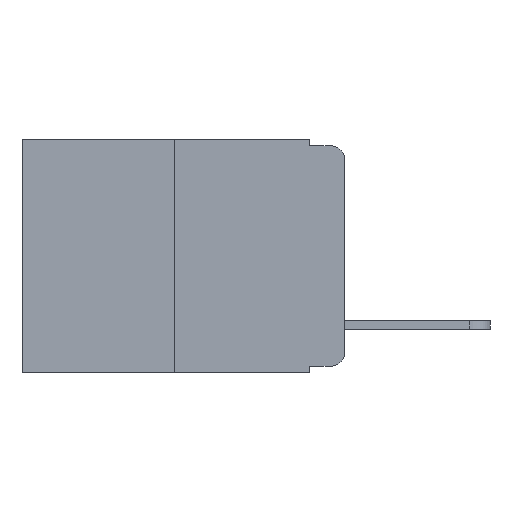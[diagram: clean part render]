
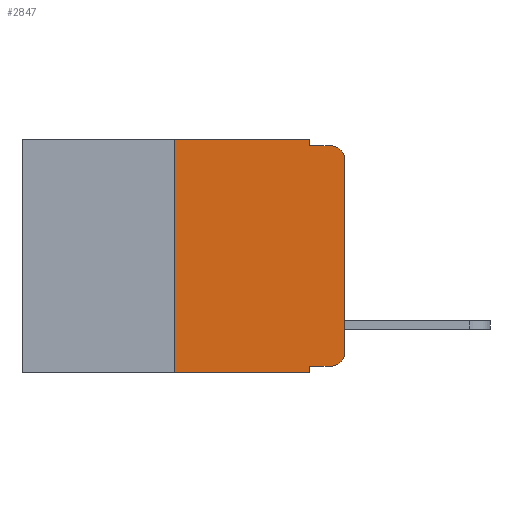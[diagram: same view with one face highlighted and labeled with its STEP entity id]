
A CAD part, left-side view. The second image highlights one B-rep face of the part: STEP entity #2847.
In plain terms, the highlighted planar face has unit normal (-1, 0, 0).
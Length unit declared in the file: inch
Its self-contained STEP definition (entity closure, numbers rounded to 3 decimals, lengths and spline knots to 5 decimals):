
#247 = PLANE ( 'NONE',  #12645 ) ;
#307 = DIRECTION ( 'NONE',  ( 0., 0., -1. ) ) ;
#566 = CARTESIAN_POINT ( 'NONE',  ( 0., 0.051, 0. ) ) ;
#1475 = EDGE_CURVE ( 'NONE', #16898, #6367, #20616, .T. ) ;
#1575 = VECTOR ( 'NONE', #20858, 39.37008 ) ;
#2296 = ORIENTED_EDGE ( 'NONE', *, *, #19439, .T. ) ;
#2613 = EDGE_CURVE ( 'NONE', #16524, #15488, #7003, .T. ) ;
#2847 = ADVANCED_FACE ( 'NONE', ( #14139 ), #247, .F. ) ;
#3010 = EDGE_LOOP ( 'NONE', ( #2296, #21992, #5674, #8573, #14335, #6886, #19723, #22819, #3377, #20828 ) ) ;
#3377 = ORIENTED_EDGE ( 'NONE', *, *, #6042, .T. ) ;
#3824 = DIRECTION ( 'NONE',  ( 1., 0., 0. ) ) ;
#3899 = CARTESIAN_POINT ( 'NONE',  ( 0., 0.473, 0. ) ) ;
#4034 = AXIS2_PLACEMENT_3D ( 'NONE', #17190, #6256, #18954 ) ;
#4114 = DIRECTION ( 'NONE',  ( 0., 0., -1. ) ) ;
#4249 = CARTESIAN_POINT ( 'NONE',  ( 0., 0.25, 0. ) ) ;
#4371 = DIRECTION ( 'NONE',  ( 0., 0., -1. ) ) ;
#4599 = CARTESIAN_POINT ( 'NONE',  ( 0., 0.051, 0. ) ) ;
#4696 = CARTESIAN_POINT ( 'NONE',  ( 0., 0.02, -0.333 ) ) ;
#5012 = CARTESIAN_POINT ( 'NONE',  ( 0., 0.051, -0.333 ) ) ;
#5510 = CARTESIAN_POINT ( 'NONE',  ( 0., 0.051, -0.343 ) ) ;
#5674 = ORIENTED_EDGE ( 'NONE', *, *, #14672, .F. ) ;
#5768 = VECTOR ( 'NONE', #14262, 39.37008 ) ;
#6014 = VECTOR ( 'NONE', #16148, 39.37008 ) ;
#6042 = EDGE_CURVE ( 'NONE', #18162, #9641, #23542, .T. ) ;
#6256 = DIRECTION ( 'NONE',  ( -1., 0., 0. ) ) ;
#6362 = VECTOR ( 'NONE', #307, 39.37008 ) ;
#6367 = VERTEX_POINT ( 'NONE', #5510 ) ;
#6886 = ORIENTED_EDGE ( 'NONE', *, *, #12231, .F. ) ;
#7003 = LINE ( 'NONE', #13521, #20836 ) ;
#7691 = VECTOR ( 'NONE', #4371, 39.37008 ) ;
#8511 = EDGE_CURVE ( 'NONE', #18162, #6367, #21948, .T. ) ;
#8573 = ORIENTED_EDGE ( 'NONE', *, *, #13457, .F. ) ;
#8756 = CARTESIAN_POINT ( 'NONE',  ( 0., 0.051, 0. ) ) ;
#8866 = CARTESIAN_POINT ( 'NONE',  ( 0., 0.25, -0.343 ) ) ;
#9131 = CARTESIAN_POINT ( 'NONE',  ( 0., 0.02, -0.03 ) ) ;
#9641 = VERTEX_POINT ( 'NONE', #4696 ) ;
#9695 = CARTESIAN_POINT ( 'NONE',  ( 0., 0.051, -0.01 ) ) ;
#11039 = DIRECTION ( 'NONE',  ( 0., 0., -1. ) ) ;
#11094 = VECTOR ( 'NONE', #21853, 39.37008 ) ;
#12142 = LINE ( 'NONE', #12144, #16405 ) ;
#12144 = CARTESIAN_POINT ( 'NONE',  ( 0., 0., 0. ) ) ;
#12231 = EDGE_CURVE ( 'NONE', #16898, #16524, #20626, .T. ) ;
#12645 = AXIS2_PLACEMENT_3D ( 'NONE', #3899, #3824, #4114 ) ;
#13457 = EDGE_CURVE ( 'NONE', #15488, #18461, #21834, .T. ) ;
#13521 = CARTESIAN_POINT ( 'NONE',  ( 0., 0.473, 0. ) ) ;
#13653 = DIRECTION ( 'NONE',  ( 0., -1., 0. ) ) ;
#13975 = DIRECTION ( 'NONE',  ( 0., 0., 1. ) ) ;
#14094 = CARTESIAN_POINT ( 'NONE',  ( 0., 0.051, -0.333 ) ) ;
#14139 = FACE_OUTER_BOUND ( 'NONE', #3010, .T. ) ;
#14262 = DIRECTION ( 'NONE',  ( 0., -1., 0. ) ) ;
#14335 = ORIENTED_EDGE ( 'NONE', *, *, #2613, .F. ) ;
#14672 = EDGE_CURVE ( 'NONE', #18461, #18626, #15785, .T. ) ;
#15488 = VERTEX_POINT ( 'NONE', #8756 ) ;
#15774 = CIRCLE ( 'NONE', #4034, 0.02 ) ;
#15785 = LINE ( 'NONE', #16197, #6014 ) ;
#16148 = DIRECTION ( 'NONE',  ( 0., -1., 0. ) ) ;
#16197 = CARTESIAN_POINT ( 'NONE',  ( 0., 0.051, -0.01 ) ) ;
#16405 = VECTOR ( 'NONE', #13975, 39.37008 ) ;
#16524 = VERTEX_POINT ( 'NONE', #4249 ) ;
#16574 = CARTESIAN_POINT ( 'NONE',  ( 0., 0., -0.03 ) ) ;
#16898 = VERTEX_POINT ( 'NONE', #8866 ) ;
#17190 = CARTESIAN_POINT ( 'NONE',  ( 0., 0.02, -0.313 ) ) ;
#17440 = CARTESIAN_POINT ( 'NONE',  ( 0., 0.02, -0.01 ) ) ;
#18162 = VERTEX_POINT ( 'NONE', #5012 ) ;
#18261 = EDGE_CURVE ( 'NONE', #22876, #18626, #20346, .T. ) ;
#18461 = VERTEX_POINT ( 'NONE', #9695 ) ;
#18626 = VERTEX_POINT ( 'NONE', #17440 ) ;
#18954 = DIRECTION ( 'NONE',  ( 0., 0., -1. ) ) ;
#19317 = CARTESIAN_POINT ( 'NONE',  ( 0., 0., -0.313 ) ) ;
#19439 = EDGE_CURVE ( 'NONE', #19905, #22876, #12142, .T. ) ;
#19723 = ORIENTED_EDGE ( 'NONE', *, *, #1475, .T. ) ;
#19905 = VERTEX_POINT ( 'NONE', #19317 ) ;
#20346 = CIRCLE ( 'NONE', #22853, 0.02 ) ;
#20616 = LINE ( 'NONE', #23212, #11094 ) ;
#20626 = LINE ( 'NONE', #20763, #1575 ) ;
#20763 = CARTESIAN_POINT ( 'NONE',  ( 0., 0.25, 0. ) ) ;
#20828 = ORIENTED_EDGE ( 'NONE', *, *, #21025, .T. ) ;
#20836 = VECTOR ( 'NONE', #13653, 39.37008 ) ;
#20858 = DIRECTION ( 'NONE',  ( 0., 0., 1. ) ) ;
#21025 = EDGE_CURVE ( 'NONE', #9641, #19905, #15774, .T. ) ;
#21653 = DIRECTION ( 'NONE',  ( -1., 0., 0. ) ) ;
#21834 = LINE ( 'NONE', #566, #6362 ) ;
#21853 = DIRECTION ( 'NONE',  ( 0., -1., 0. ) ) ;
#21948 = LINE ( 'NONE', #4599, #7691 ) ;
#21992 = ORIENTED_EDGE ( 'NONE', *, *, #18261, .T. ) ;
#22819 = ORIENTED_EDGE ( 'NONE', *, *, #8511, .F. ) ;
#22853 = AXIS2_PLACEMENT_3D ( 'NONE', #9131, #21653, #11039 ) ;
#22876 = VERTEX_POINT ( 'NONE', #16574 ) ;
#23212 = CARTESIAN_POINT ( 'NONE',  ( 0., 0.473, -0.343 ) ) ;
#23542 = LINE ( 'NONE', #14094, #5768 ) ;
